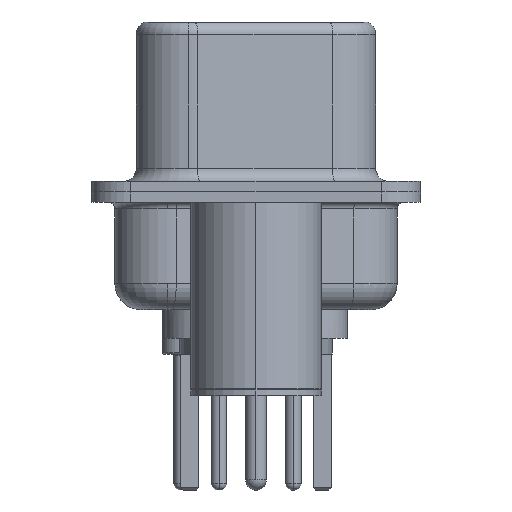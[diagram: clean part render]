
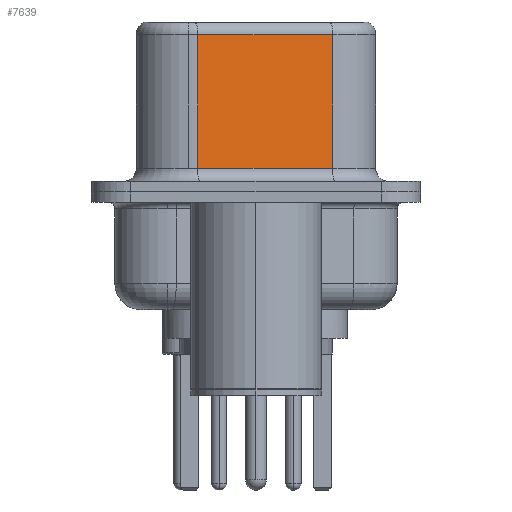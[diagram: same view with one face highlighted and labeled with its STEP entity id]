
A CAD part, left-side view. The second image highlights one B-rep face of the part: STEP entity #7639.
In plain terms, the highlighted planar face has unit normal (-0.985, -0.174, 0).
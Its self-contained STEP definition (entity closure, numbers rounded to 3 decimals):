
#491 = CARTESIAN_POINT ( 'NONE',  ( 3.675, 2.233, 6.02 ) ) ;
#1805 = VECTOR ( 'NONE', #19065, 1000. ) ;
#3487 = ORIENTED_EDGE ( 'NONE', *, *, #18397, .T. ) ;
#3644 = CARTESIAN_POINT ( 'NONE',  ( 4.585, -2.927, 6.52 ) ) ;
#4711 = VECTOR ( 'NONE', #11562, 1000. ) ;
#5648 = VECTOR ( 'NONE', #8673, 1000. ) ;
#5773 = LINE ( 'NONE', #12262, #20063 ) ;
#7533 = DIRECTION ( 'NONE',  ( 0.985, 0.174, 0. ) ) ;
#7639 = ADVANCED_FACE ( 'NONE', ( #16307 ), #9055, .F. ) ;
#7803 = EDGE_LOOP ( 'NONE', ( #14337, #20776, #19273, #3487 ) ) ;
#8673 = DIRECTION ( 'NONE',  ( 0., 0., -1. ) ) ;
#8821 = CARTESIAN_POINT ( 'NONE',  ( 4.585, -2.927, 6.52 ) ) ;
#9055 = PLANE ( 'NONE',  #21529 ) ;
#10418 = DIRECTION ( 'NONE',  ( 0.174, -0.985, 0. ) ) ;
#11051 = LINE ( 'NONE', #19206, #4711 ) ;
#11562 = DIRECTION ( 'NONE',  ( -0.174, 0.985, 0. ) ) ;
#12185 = CARTESIAN_POINT ( 'NONE',  ( 4.585, -2.927, 6.02 ) ) ;
#12262 = CARTESIAN_POINT ( 'NONE',  ( 4.585, -2.927, 0.9 ) ) ;
#13980 = LINE ( 'NONE', #8821, #5648 ) ;
#14337 = ORIENTED_EDGE ( 'NONE', *, *, #21330, .F. ) ;
#14971 = DIRECTION ( 'NONE',  ( -0.174, 0.985, 0. ) ) ;
#16033 = CARTESIAN_POINT ( 'NONE',  ( 4.585, -2.927, 0.9 ) ) ;
#16194 = VERTEX_POINT ( 'NONE', #491 ) ;
#16307 = FACE_OUTER_BOUND ( 'NONE', #7803, .T. ) ;
#16511 = LINE ( 'NONE', #22571, #1805 ) ;
#18397 = EDGE_CURVE ( 'NONE', #21759, #19299, #5773, .T. ) ;
#18599 = CARTESIAN_POINT ( 'NONE',  ( 3.675, 2.233, 0.9 ) ) ;
#19065 = DIRECTION ( 'NONE',  ( 0., 0., -1. ) ) ;
#19206 = CARTESIAN_POINT ( 'NONE',  ( 4.585, -2.927, 6.02 ) ) ;
#19273 = ORIENTED_EDGE ( 'NONE', *, *, #22968, .T. ) ;
#19299 = VERTEX_POINT ( 'NONE', #16033 ) ;
#20063 = VECTOR ( 'NONE', #10418, 1000. ) ;
#20776 = ORIENTED_EDGE ( 'NONE', *, *, #23025, .T. ) ;
#21233 = VERTEX_POINT ( 'NONE', #12185 ) ;
#21330 = EDGE_CURVE ( 'NONE', #21233, #19299, #13980, .T. ) ;
#21529 = AXIS2_PLACEMENT_3D ( 'NONE', #3644, #7533, #14971 ) ;
#21759 = VERTEX_POINT ( 'NONE', #18599 ) ;
#22571 = CARTESIAN_POINT ( 'NONE',  ( 3.675, 2.233, 6.52 ) ) ;
#22968 = EDGE_CURVE ( 'NONE', #16194, #21759, #16511, .T. ) ;
#23025 = EDGE_CURVE ( 'NONE', #21233, #16194, #11051, .T. ) ;
